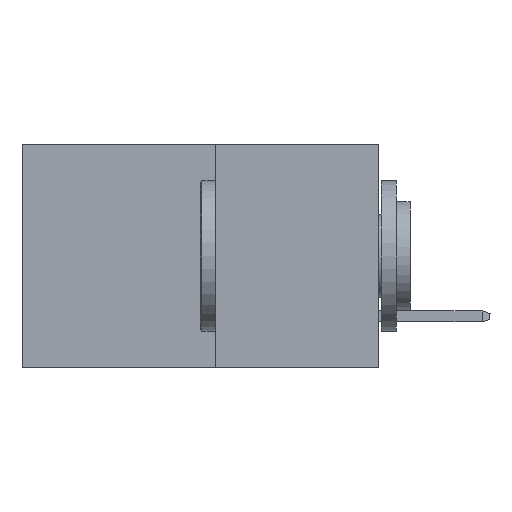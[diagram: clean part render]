
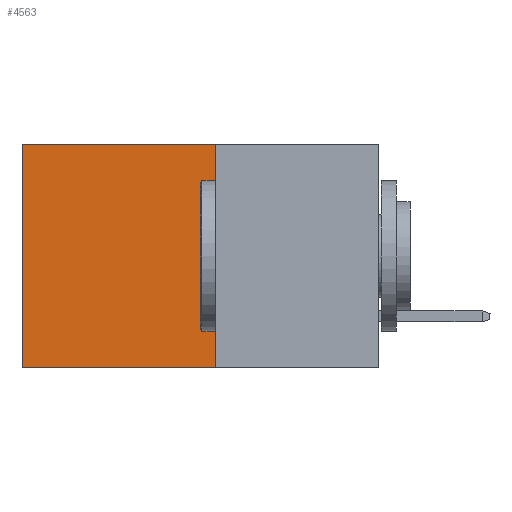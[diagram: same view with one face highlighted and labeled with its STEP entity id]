
A CAD part, left-side view. The second image highlights one B-rep face of the part: STEP entity #4563.
In plain terms, the highlighted planar face has unit normal (-1, 0, 0).
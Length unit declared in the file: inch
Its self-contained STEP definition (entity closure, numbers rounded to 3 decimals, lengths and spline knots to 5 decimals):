
#13 = ORIENTED_EDGE ( 'NONE', *, *, #16397, .T. ) ;
#284 = ORIENTED_EDGE ( 'NONE', *, *, #12721, .F. ) ;
#418 = DIRECTION ( 'NONE',  ( 0., 0., -1. ) ) ;
#957 = CARTESIAN_POINT ( 'NONE',  ( 0.277, 0.27, 0. ) ) ;
#1011 = DIRECTION ( 'NONE',  ( 0., 1., 0. ) ) ;
#1488 = DIRECTION ( 'NONE',  ( 1., 0., 0. ) ) ;
#1557 = CARTESIAN_POINT ( 'NONE',  ( 0.277, 0.27, -0.37 ) ) ;
#1563 = PLANE ( 'NONE',  #8638 ) ;
#1581 = VERTEX_POINT ( 'NONE', #6471 ) ;
#2039 = CARTESIAN_POINT ( 'NONE',  ( 0.277, 0.59, 0. ) ) ;
#4518 = ORIENTED_EDGE ( 'NONE', *, *, #9174, .T. ) ;
#4563 = ADVANCED_FACE ( 'NONE', ( #5631 ), #1563, .F. ) ;
#4586 = CARTESIAN_POINT ( 'NONE',  ( 0.277, 0.59, -0.37 ) ) ;
#5554 = DIRECTION ( 'NONE',  ( 0., 0., -1. ) ) ;
#5631 = FACE_OUTER_BOUND ( 'NONE', #11897, .T. ) ;
#5799 = LINE ( 'NONE', #11113, #17690 ) ;
#6471 = CARTESIAN_POINT ( 'NONE',  ( 0.277, 0.27, -0.37 ) ) ;
#7620 = LINE ( 'NONE', #19466, #19383 ) ;
#8473 = CARTESIAN_POINT ( 'NONE',  ( 0.277, 0.27, -0.37 ) ) ;
#8638 = AXIS2_PLACEMENT_3D ( 'NONE', #1557, #1488, #418 ) ;
#9174 = EDGE_CURVE ( 'NONE', #16420, #16853, #5799, .T. ) ;
#10656 = LINE ( 'NONE', #13414, #11653 ) ;
#11091 = DIRECTION ( 'NONE',  ( 0., 1., 0. ) ) ;
#11113 = CARTESIAN_POINT ( 'NONE',  ( 0.277, 0.27, 0. ) ) ;
#11653 = VECTOR ( 'NONE', #5554, 39.37008 ) ;
#11835 = VECTOR ( 'NONE', #17728, 39.37008 ) ;
#11897 = EDGE_LOOP ( 'NONE', ( #13, #17508, #284, #4518 ) ) ;
#12180 = EDGE_CURVE ( 'NONE', #1581, #17181, #7620, .T. ) ;
#12721 = EDGE_CURVE ( 'NONE', #16420, #1581, #19819, .T. ) ;
#13414 = CARTESIAN_POINT ( 'NONE',  ( 0.277, 0.59, -0.37 ) ) ;
#16397 = EDGE_CURVE ( 'NONE', #16853, #17181, #10656, .T. ) ;
#16420 = VERTEX_POINT ( 'NONE', #957 ) ;
#16853 = VERTEX_POINT ( 'NONE', #2039 ) ;
#17181 = VERTEX_POINT ( 'NONE', #4586 ) ;
#17508 = ORIENTED_EDGE ( 'NONE', *, *, #12180, .F. ) ;
#17690 = VECTOR ( 'NONE', #11091, 39.37008 ) ;
#17728 = DIRECTION ( 'NONE',  ( 0., 0., -1. ) ) ;
#19383 = VECTOR ( 'NONE', #1011, 39.37008 ) ;
#19466 = CARTESIAN_POINT ( 'NONE',  ( 0.277, 0.27, -0.37 ) ) ;
#19819 = LINE ( 'NONE', #8473, #11835 ) ;
